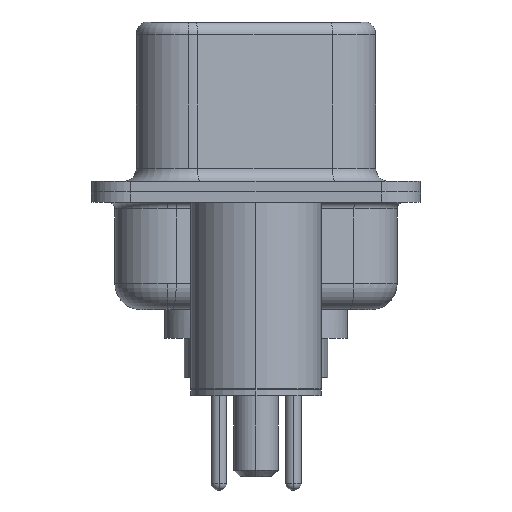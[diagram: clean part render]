
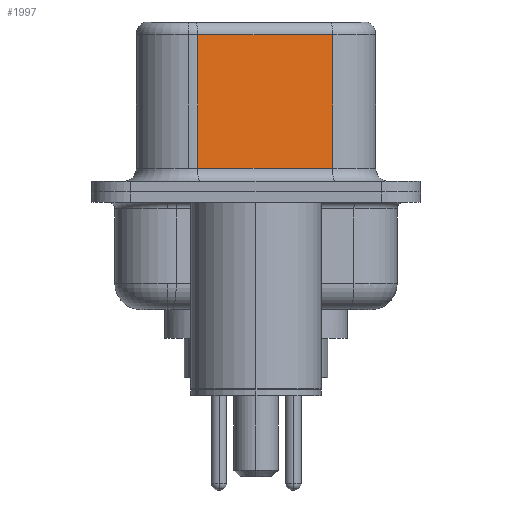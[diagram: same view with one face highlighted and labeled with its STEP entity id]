
A CAD part, left-side view. The second image highlights one B-rep face of the part: STEP entity #1997.
In plain terms, the highlighted planar face has unit normal (-0.985, -0.174, 0).
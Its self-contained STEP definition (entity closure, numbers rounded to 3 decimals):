
#248 = ORIENTED_EDGE ( 'NONE', *, *, #6536, .T. ) ;
#338 = DIRECTION ( 'NONE',  ( 0.985, 0.174, 0. ) ) ;
#419 = VECTOR ( 'NONE', #10686, 1000. ) ;
#479 = DIRECTION ( 'NONE',  ( 0., 0., -1. ) ) ;
#581 = CARTESIAN_POINT ( 'NONE',  ( 4.58, -2.927, 6.52 ) ) ;
#1312 = EDGE_LOOP ( 'NONE', ( #8172, #248, #9595, #13793 ) ) ;
#1635 = DIRECTION ( 'NONE',  ( -0.174, 0.985, 0. ) ) ;
#1997 = ADVANCED_FACE ( 'NONE', ( #9123 ), #4987, .F. ) ;
#2149 = LINE ( 'NONE', #7244, #13112 ) ;
#2168 = CARTESIAN_POINT ( 'NONE',  ( 3.67, 2.233, 0.9 ) ) ;
#2362 = CARTESIAN_POINT ( 'NONE',  ( 3.67, 2.233, 6.52 ) ) ;
#2840 = CARTESIAN_POINT ( 'NONE',  ( 4.58, -2.927, 0.9 ) ) ;
#3764 = VECTOR ( 'NONE', #479, 1000. ) ;
#4373 = VERTEX_POINT ( 'NONE', #2168 ) ;
#4987 = PLANE ( 'NONE',  #6231 ) ;
#5569 = VERTEX_POINT ( 'NONE', #10582 ) ;
#6231 = AXIS2_PLACEMENT_3D ( 'NONE', #581, #338, #10999 ) ;
#6536 = EDGE_CURVE ( 'NONE', #10443, #8260, #2149, .T. ) ;
#6771 = LINE ( 'NONE', #8309, #3764 ) ;
#6935 = CARTESIAN_POINT ( 'NONE',  ( 4.58, -2.927, 6.02 ) ) ;
#7244 = CARTESIAN_POINT ( 'NONE',  ( 4.58, -2.927, 6.02 ) ) ;
#8172 = ORIENTED_EDGE ( 'NONE', *, *, #9290, .F. ) ;
#8260 = VERTEX_POINT ( 'NONE', #14505 ) ;
#8309 = CARTESIAN_POINT ( 'NONE',  ( 4.58, -2.927, 6.52 ) ) ;
#9039 = LINE ( 'NONE', #2840, #419 ) ;
#9123 = FACE_OUTER_BOUND ( 'NONE', #1312, .T. ) ;
#9290 = EDGE_CURVE ( 'NONE', #10443, #5569, #6771, .T. ) ;
#9328 = EDGE_CURVE ( 'NONE', #4373, #5569, #9039, .T. ) ;
#9595 = ORIENTED_EDGE ( 'NONE', *, *, #9974, .T. ) ;
#9974 = EDGE_CURVE ( 'NONE', #8260, #4373, #13119, .T. ) ;
#10088 = VECTOR ( 'NONE', #11383, 1000. ) ;
#10443 = VERTEX_POINT ( 'NONE', #6935 ) ;
#10582 = CARTESIAN_POINT ( 'NONE',  ( 4.58, -2.927, 0.9 ) ) ;
#10686 = DIRECTION ( 'NONE',  ( 0.174, -0.985, 0. ) ) ;
#10999 = DIRECTION ( 'NONE',  ( -0.174, 0.985, 0. ) ) ;
#11383 = DIRECTION ( 'NONE',  ( 0., 0., -1. ) ) ;
#13112 = VECTOR ( 'NONE', #1635, 1000. ) ;
#13119 = LINE ( 'NONE', #2362, #10088 ) ;
#13793 = ORIENTED_EDGE ( 'NONE', *, *, #9328, .T. ) ;
#14505 = CARTESIAN_POINT ( 'NONE',  ( 3.67, 2.233, 6.02 ) ) ;
